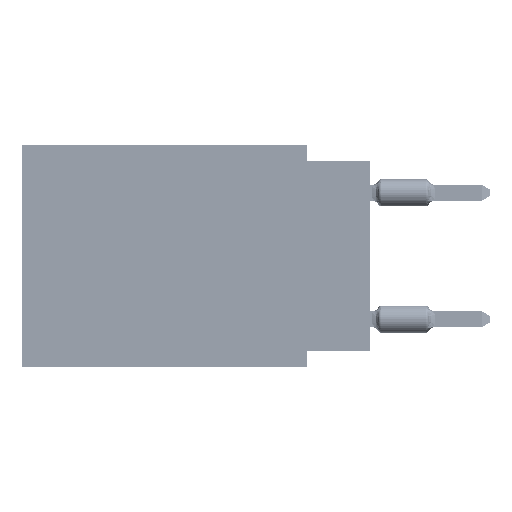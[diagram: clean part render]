
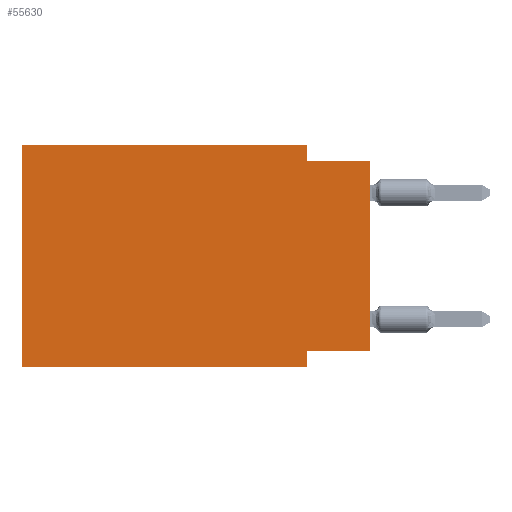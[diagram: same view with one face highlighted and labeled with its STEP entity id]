
A CAD part, left-side view. The second image highlights one B-rep face of the part: STEP entity #55630.
In plain terms, the highlighted planar face has unit normal (-1, 0, 0).
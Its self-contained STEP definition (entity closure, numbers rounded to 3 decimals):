
#3711 = ORIENTED_EDGE ( 'NONE', *, *, #45092, .F. ) ;
#4827 = CARTESIAN_POINT ( 'NONE',  ( 0., 13.97, 0. ) ) ;
#12215 = EDGE_CURVE ( 'NONE', #23945, #85245, #111996, .T. ) ;
#12574 = VECTOR ( 'NONE', #74462, 1000. ) ;
#13387 = LINE ( 'NONE', #4827, #92763 ) ;
#15026 = VERTEX_POINT ( 'NONE', #57898 ) ;
#15099 = LINE ( 'NONE', #91892, #41675 ) ;
#15983 = EDGE_CURVE ( 'NONE', #71926, #85245, #39199, .T. ) ;
#23658 = VECTOR ( 'NONE', #68733, 1000. ) ;
#23937 = EDGE_CURVE ( 'NONE', #79341, #23945, #83913, .T. ) ;
#23945 = VERTEX_POINT ( 'NONE', #111727 ) ;
#24117 = CARTESIAN_POINT ( 'NONE',  ( 0., 0., -0.635 ) ) ;
#24445 = DIRECTION ( 'NONE',  ( 0., -1., 0. ) ) ;
#25227 = CARTESIAN_POINT ( 'NONE',  ( 0., 13.97, -8.89 ) ) ;
#26063 = ORIENTED_EDGE ( 'NONE', *, *, #12215, .F. ) ;
#28432 = AXIS2_PLACEMENT_3D ( 'NONE', #33224, #67903, #85517 ) ;
#28994 = EDGE_CURVE ( 'NONE', #34595, #29673, #15099, .T. ) ;
#29673 = VERTEX_POINT ( 'NONE', #70599 ) ;
#33224 = CARTESIAN_POINT ( 'NONE',  ( 0., 13.97, 0. ) ) ;
#34043 = CARTESIAN_POINT ( 'NONE',  ( 0., 13.97, 0. ) ) ;
#34595 = VERTEX_POINT ( 'NONE', #25227 ) ;
#34740 = CARTESIAN_POINT ( 'NONE',  ( 0., 0., -8.255 ) ) ;
#39199 = LINE ( 'NONE', #99458, #50698 ) ;
#40157 = DIRECTION ( 'NONE',  ( 0., -1., 0. ) ) ;
#41675 = VECTOR ( 'NONE', #40157, 1000. ) ;
#42793 = EDGE_LOOP ( 'NONE', ( #104999, #26063, #75928, #85914, #91794, #94134, #53989, #3711 ) ) ;
#43917 = EDGE_CURVE ( 'NONE', #59491, #29673, #110239, .T. ) ;
#45092 = EDGE_CURVE ( 'NONE', #71926, #59491, #94291, .T. ) ;
#46920 = DIRECTION ( 'NONE',  ( 0., -1., 0. ) ) ;
#48858 = CARTESIAN_POINT ( 'NONE',  ( 0., 0., -8.255 ) ) ;
#49501 = VECTOR ( 'NONE', #24445, 1000. ) ;
#49625 = CARTESIAN_POINT ( 'NONE',  ( 0., 2.54, -8.255 ) ) ;
#50698 = VECTOR ( 'NONE', #90359, 1000. ) ;
#51397 = FACE_OUTER_BOUND ( 'NONE', #42793, .T. ) ;
#53989 = ORIENTED_EDGE ( 'NONE', *, *, #43917, .F. ) ;
#55630 = ADVANCED_FACE ( 'NONE', ( #51397 ), #86068, .F. ) ;
#56333 = VECTOR ( 'NONE', #93741, 1000. ) ;
#57898 = CARTESIAN_POINT ( 'NONE',  ( 0., 13.97, 0. ) ) ;
#57926 = CARTESIAN_POINT ( 'NONE',  ( 0., 2.54, -8.89 ) ) ;
#59390 = DIRECTION ( 'NONE',  ( 0., 0., -1. ) ) ;
#59491 = VERTEX_POINT ( 'NONE', #49625 ) ;
#67903 = DIRECTION ( 'NONE',  ( 1., 0., 0. ) ) ;
#68733 = DIRECTION ( 'NONE',  ( 0., 0., 1. ) ) ;
#70599 = CARTESIAN_POINT ( 'NONE',  ( 0., 2.54, -8.89 ) ) ;
#71926 = VERTEX_POINT ( 'NONE', #34740 ) ;
#74462 = DIRECTION ( 'NONE',  ( 0., 0., -1. ) ) ;
#75397 = VECTOR ( 'NONE', #59390, 1000. ) ;
#75928 = ORIENTED_EDGE ( 'NONE', *, *, #23937, .F. ) ;
#79341 = VERTEX_POINT ( 'NONE', #85337 ) ;
#83913 = LINE ( 'NONE', #110619, #75397 ) ;
#85245 = VERTEX_POINT ( 'NONE', #24117 ) ;
#85337 = CARTESIAN_POINT ( 'NONE',  ( 0., 2.54, 0. ) ) ;
#85517 = DIRECTION ( 'NONE',  ( 0., 0., -1. ) ) ;
#85914 = ORIENTED_EDGE ( 'NONE', *, *, #87025, .F. ) ;
#86068 = PLANE ( 'NONE',  #28432 ) ;
#86271 = EDGE_CURVE ( 'NONE', #34595, #15026, #111951, .T. ) ;
#87025 = EDGE_CURVE ( 'NONE', #15026, #79341, #13387, .T. ) ;
#90359 = DIRECTION ( 'NONE',  ( 0., 0., 1. ) ) ;
#91794 = ORIENTED_EDGE ( 'NONE', *, *, #86271, .F. ) ;
#91892 = CARTESIAN_POINT ( 'NONE',  ( 0., 13.97, -8.89 ) ) ;
#92763 = VECTOR ( 'NONE', #46920, 1000. ) ;
#93741 = DIRECTION ( 'NONE',  ( 0., 1., 0. ) ) ;
#94134 = ORIENTED_EDGE ( 'NONE', *, *, #28994, .T. ) ;
#94291 = LINE ( 'NONE', #48858, #56333 ) ;
#99458 = CARTESIAN_POINT ( 'NONE',  ( 0., 0., 0. ) ) ;
#104999 = ORIENTED_EDGE ( 'NONE', *, *, #15983, .T. ) ;
#110239 = LINE ( 'NONE', #57926, #12574 ) ;
#110619 = CARTESIAN_POINT ( 'NONE',  ( 0., 2.54, 0. ) ) ;
#110904 = CARTESIAN_POINT ( 'NONE',  ( 0., 0., -0.635 ) ) ;
#111727 = CARTESIAN_POINT ( 'NONE',  ( 0., 2.54, -0.635 ) ) ;
#111951 = LINE ( 'NONE', #34043, #23658 ) ;
#111996 = LINE ( 'NONE', #110904, #49501 ) ;
